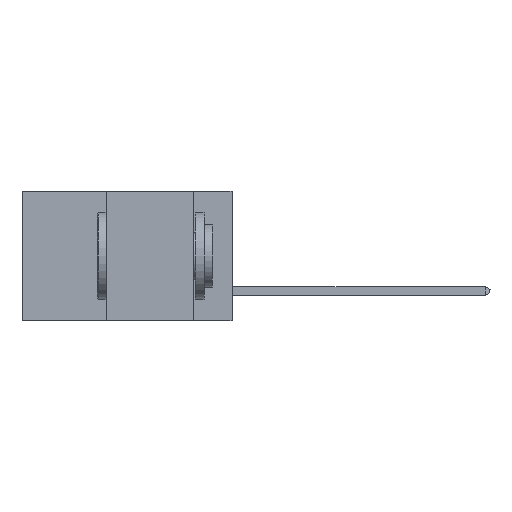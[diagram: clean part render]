
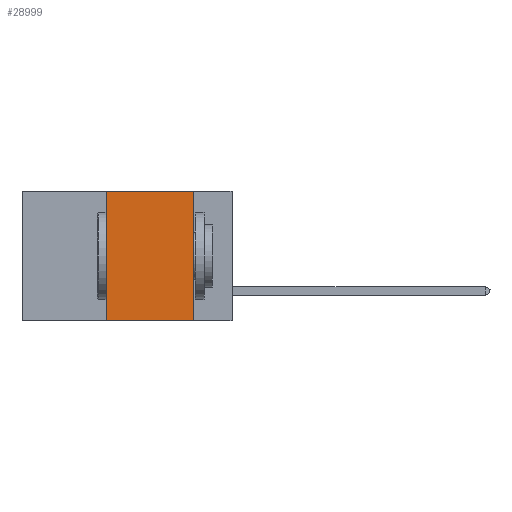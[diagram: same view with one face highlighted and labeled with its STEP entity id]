
A CAD part, left-side view. The second image highlights one B-rep face of the part: STEP entity #28999.
In plain terms, the highlighted planar face has unit normal (-1, 0, 0).
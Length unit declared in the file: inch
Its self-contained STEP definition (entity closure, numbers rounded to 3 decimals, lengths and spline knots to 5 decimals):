
#187 = EDGE_CURVE ( 'NONE', #22743, #13805, #15621, .T. ) ;
#372 = ORIENTED_EDGE ( 'NONE', *, *, #187, .F. ) ;
#1977 = VECTOR ( 'NONE', #5387, 39.37008 ) ;
#4321 = DIRECTION ( 'NONE',  ( 0., 0., -1. ) ) ;
#4987 = DIRECTION ( 'NONE',  ( 0., 0., 1. ) ) ;
#5387 = DIRECTION ( 'NONE',  ( 0., -1., 0. ) ) ;
#5459 = VERTEX_POINT ( 'NONE', #23625 ) ;
#5539 = LINE ( 'NONE', #27410, #25948 ) ;
#5911 = ORIENTED_EDGE ( 'NONE', *, *, #12853, .T. ) ;
#6681 = LINE ( 'NONE', #20042, #28157 ) ;
#8426 = EDGE_LOOP ( 'NONE', ( #21810, #372, #21924, #5911 ) ) ;
#8583 = DIRECTION ( 'NONE',  ( 1., 0., 0. ) ) ;
#9838 = CARTESIAN_POINT ( 'NONE',  ( 0., 0.6, 0. ) ) ;
#10315 = CARTESIAN_POINT ( 'NONE',  ( 0., 0.11, -0.37 ) ) ;
#11046 = DIRECTION ( 'NONE',  ( 0., 0., -1. ) ) ;
#12361 = AXIS2_PLACEMENT_3D ( 'NONE', #28929, #8583, #4321 ) ;
#12853 = EDGE_CURVE ( 'NONE', #5459, #13922, #20829, .T. ) ;
#12968 = PLANE ( 'NONE',  #12361 ) ;
#13150 = DIRECTION ( 'NONE',  ( 0., -1., 0. ) ) ;
#13476 = CARTESIAN_POINT ( 'NONE',  ( 0., 0.6, -0.37 ) ) ;
#13805 = VERTEX_POINT ( 'NONE', #14187 ) ;
#13922 = VERTEX_POINT ( 'NONE', #10315 ) ;
#14187 = CARTESIAN_POINT ( 'NONE',  ( 0., 0.11, 0. ) ) ;
#15621 = LINE ( 'NONE', #9838, #1977 ) ;
#15842 = EDGE_CURVE ( 'NONE', #5459, #22743, #5539, .T. ) ;
#18024 = CARTESIAN_POINT ( 'NONE',  ( 0., 0.36, 0. ) ) ;
#18071 = VECTOR ( 'NONE', #13150, 39.37008 ) ;
#20031 = FACE_OUTER_BOUND ( 'NONE', #8426, .T. ) ;
#20042 = CARTESIAN_POINT ( 'NONE',  ( 0., 0.11, 0. ) ) ;
#20829 = LINE ( 'NONE', #13476, #18071 ) ;
#21810 = ORIENTED_EDGE ( 'NONE', *, *, #28984, .F. ) ;
#21924 = ORIENTED_EDGE ( 'NONE', *, *, #15842, .F. ) ;
#22743 = VERTEX_POINT ( 'NONE', #18024 ) ;
#23625 = CARTESIAN_POINT ( 'NONE',  ( 0., 0.36, -0.37 ) ) ;
#25948 = VECTOR ( 'NONE', #4987, 39.37008 ) ;
#27410 = CARTESIAN_POINT ( 'NONE',  ( 0., 0.36, 0. ) ) ;
#28157 = VECTOR ( 'NONE', #11046, 39.37008 ) ;
#28929 = CARTESIAN_POINT ( 'NONE',  ( 0., 0.6, 0. ) ) ;
#28984 = EDGE_CURVE ( 'NONE', #13805, #13922, #6681, .T. ) ;
#28999 = ADVANCED_FACE ( 'NONE', ( #20031 ), #12968, .F. ) ;
